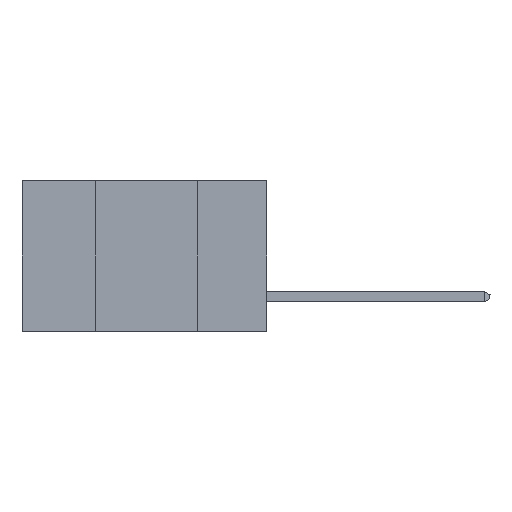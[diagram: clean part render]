
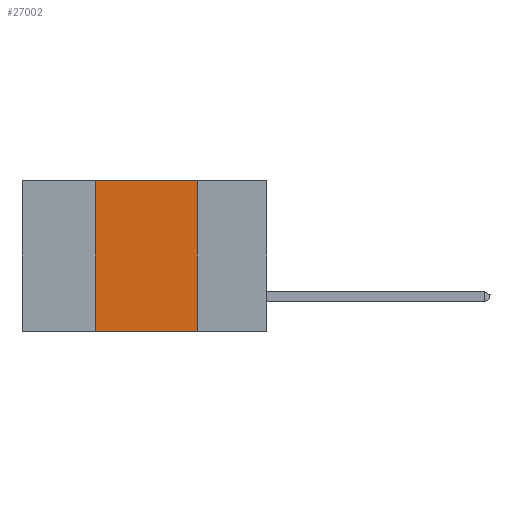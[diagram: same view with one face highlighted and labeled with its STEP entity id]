
A CAD part, left-side view. The second image highlights one B-rep face of the part: STEP entity #27002.
In plain terms, the highlighted planar face has unit normal (-1, 0, 0).
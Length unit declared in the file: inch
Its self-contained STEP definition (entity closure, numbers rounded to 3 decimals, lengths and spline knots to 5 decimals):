
#1508 = LINE ( 'NONE', #15393, #2369 ) ;
#2326 = CARTESIAN_POINT ( 'NONE',  ( 0., 0.42, 0. ) ) ;
#2369 = VECTOR ( 'NONE', #7383, 39.37008 ) ;
#4882 = EDGE_CURVE ( 'NONE', #17054, #19560, #18885, .T. ) ;
#5193 = VECTOR ( 'NONE', #11611, 39.37008 ) ;
#6801 = CARTESIAN_POINT ( 'NONE',  ( 0., 0.42, -0.37 ) ) ;
#7383 = DIRECTION ( 'NONE',  ( 0., -1., 0. ) ) ;
#7741 = EDGE_CURVE ( 'NONE', #9481, #33641, #20756, .T. ) ;
#8125 = AXIS2_PLACEMENT_3D ( 'NONE', #26786, #12765, #10498 ) ;
#9481 = VERTEX_POINT ( 'NONE', #6801 ) ;
#10498 = DIRECTION ( 'NONE',  ( 0., 0., -1. ) ) ;
#11611 = DIRECTION ( 'NONE',  ( 0., 0., -1. ) ) ;
#12236 = ORIENTED_EDGE ( 'NONE', *, *, #21931, .F. ) ;
#12765 = DIRECTION ( 'NONE',  ( 1., 0., 0. ) ) ;
#13092 = DIRECTION ( 'NONE',  ( 0., 0., 1. ) ) ;
#13541 = ORIENTED_EDGE ( 'NONE', *, *, #4882, .F. ) ;
#13608 = EDGE_LOOP ( 'NONE', ( #13541, #12236, #18303, #20526 ) ) ;
#14157 = FACE_OUTER_BOUND ( 'NONE', #13608, .T. ) ;
#14197 = EDGE_CURVE ( 'NONE', #9481, #19560, #1508, .T. ) ;
#15393 = CARTESIAN_POINT ( 'NONE',  ( 0., 0.6, -0.37 ) ) ;
#17054 = VERTEX_POINT ( 'NONE', #32797 ) ;
#18303 = ORIENTED_EDGE ( 'NONE', *, *, #7741, .F. ) ;
#18885 = LINE ( 'NONE', #28184, #5193 ) ;
#19560 = VERTEX_POINT ( 'NONE', #25568 ) ;
#20526 = ORIENTED_EDGE ( 'NONE', *, *, #14197, .T. ) ;
#20756 = LINE ( 'NONE', #2326, #27151 ) ;
#21740 = DIRECTION ( 'NONE',  ( 0., -1., 0. ) ) ;
#21931 = EDGE_CURVE ( 'NONE', #33641, #17054, #24349, .T. ) ;
#23509 = VECTOR ( 'NONE', #21740, 39.37008 ) ;
#24349 = LINE ( 'NONE', #27115, #23509 ) ;
#25568 = CARTESIAN_POINT ( 'NONE',  ( 0., 0.17, -0.37 ) ) ;
#26786 = CARTESIAN_POINT ( 'NONE',  ( 0., 0.6, 0. ) ) ;
#27002 = ADVANCED_FACE ( 'NONE', ( #14157 ), #29224, .F. ) ;
#27115 = CARTESIAN_POINT ( 'NONE',  ( 0., 0.6, 0. ) ) ;
#27151 = VECTOR ( 'NONE', #13092, 39.37008 ) ;
#27774 = CARTESIAN_POINT ( 'NONE',  ( 0., 0.42, 0. ) ) ;
#28184 = CARTESIAN_POINT ( 'NONE',  ( 0., 0.17, 0. ) ) ;
#29224 = PLANE ( 'NONE',  #8125 ) ;
#32797 = CARTESIAN_POINT ( 'NONE',  ( 0., 0.17, 0. ) ) ;
#33641 = VERTEX_POINT ( 'NONE', #27774 ) ;
